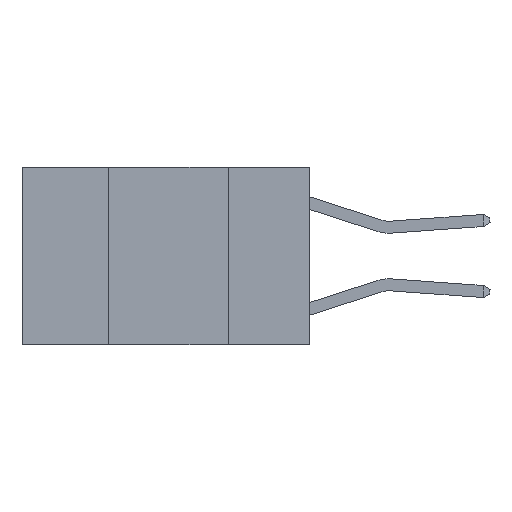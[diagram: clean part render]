
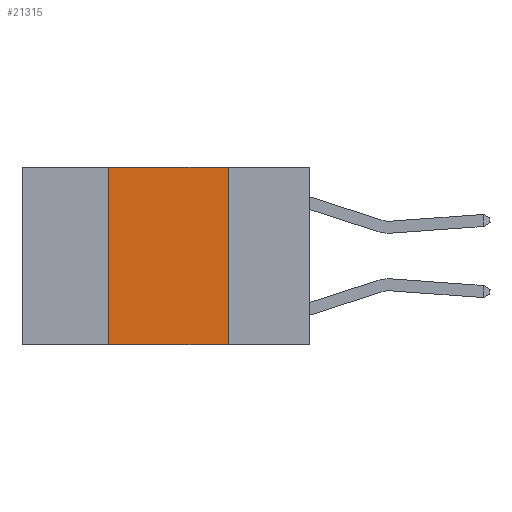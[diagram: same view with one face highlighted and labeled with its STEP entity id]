
A CAD part, left-side view. The second image highlights one B-rep face of the part: STEP entity #21315.
In plain terms, the highlighted planar face has unit normal (-1, 0, 0).
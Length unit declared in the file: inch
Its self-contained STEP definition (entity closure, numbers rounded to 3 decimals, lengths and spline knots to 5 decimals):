
#166 = CARTESIAN_POINT ( 'NONE',  ( 0., 0.6, -0.37 ) ) ;
#1783 = ORIENTED_EDGE ( 'NONE', *, *, #13210, .F. ) ;
#2402 = AXIS2_PLACEMENT_3D ( 'NONE', #4410, #6072, #21951 ) ;
#4410 = CARTESIAN_POINT ( 'NONE',  ( 0., 0.6, 0. ) ) ;
#6031 = LINE ( 'NONE', #15160, #19867 ) ;
#6072 = DIRECTION ( 'NONE',  ( 1., 0., 0. ) ) ;
#6953 = VERTEX_POINT ( 'NONE', #13260 ) ;
#7910 = ORIENTED_EDGE ( 'NONE', *, *, #21745, .F. ) ;
#8286 = CARTESIAN_POINT ( 'NONE',  ( 0., 0.42, -0.37 ) ) ;
#8606 = LINE ( 'NONE', #17737, #22125 ) ;
#8982 = LINE ( 'NONE', #17953, #29104 ) ;
#9213 = VERTEX_POINT ( 'NONE', #24067 ) ;
#10424 = LINE ( 'NONE', #166, #10987 ) ;
#10987 = VECTOR ( 'NONE', #15389, 39.37008 ) ;
#12631 = EDGE_CURVE ( 'NONE', #22531, #24005, #8606, .T. ) ;
#13129 = PLANE ( 'NONE',  #2402 ) ;
#13210 = EDGE_CURVE ( 'NONE', #24005, #9213, #8982, .T. ) ;
#13260 = CARTESIAN_POINT ( 'NONE',  ( 0., 0.17, -0.37 ) ) ;
#13307 = DIRECTION ( 'NONE',  ( 0., 0., 1. ) ) ;
#13396 = ORIENTED_EDGE ( 'NONE', *, *, #22192, .T. ) ;
#15160 = CARTESIAN_POINT ( 'NONE',  ( 0., 0.17, 0. ) ) ;
#15389 = DIRECTION ( 'NONE',  ( 0., -1., 0. ) ) ;
#17737 = CARTESIAN_POINT ( 'NONE',  ( 0., 0.42, 0. ) ) ;
#17953 = CARTESIAN_POINT ( 'NONE',  ( 0., 0.6, 0. ) ) ;
#18894 = ORIENTED_EDGE ( 'NONE', *, *, #12631, .F. ) ;
#19637 = CARTESIAN_POINT ( 'NONE',  ( 0., 0.42, 0. ) ) ;
#19867 = VECTOR ( 'NONE', #26603, 39.37008 ) ;
#21315 = ADVANCED_FACE ( 'NONE', ( #24147 ), #13129, .F. ) ;
#21745 = EDGE_CURVE ( 'NONE', #9213, #6953, #6031, .T. ) ;
#21951 = DIRECTION ( 'NONE',  ( 0., 0., -1. ) ) ;
#22125 = VECTOR ( 'NONE', #13307, 39.37008 ) ;
#22192 = EDGE_CURVE ( 'NONE', #22531, #6953, #10424, .T. ) ;
#22531 = VERTEX_POINT ( 'NONE', #8286 ) ;
#24005 = VERTEX_POINT ( 'NONE', #19637 ) ;
#24067 = CARTESIAN_POINT ( 'NONE',  ( 0., 0.17, 0. ) ) ;
#24147 = FACE_OUTER_BOUND ( 'NONE', #28249, .T. ) ;
#26603 = DIRECTION ( 'NONE',  ( 0., 0., -1. ) ) ;
#26895 = DIRECTION ( 'NONE',  ( 0., -1., 0. ) ) ;
#28249 = EDGE_LOOP ( 'NONE', ( #7910, #1783, #18894, #13396 ) ) ;
#29104 = VECTOR ( 'NONE', #26895, 39.37008 ) ;
